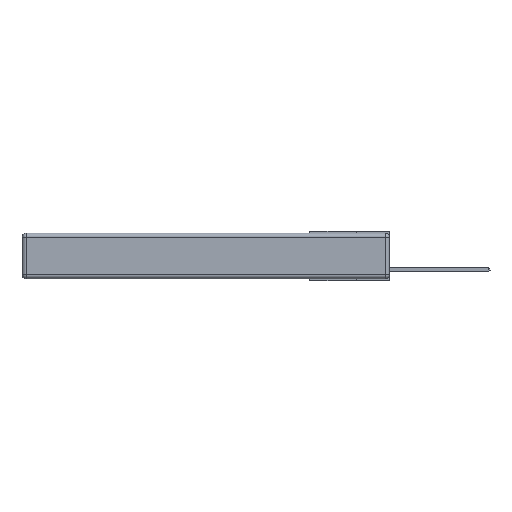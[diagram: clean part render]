
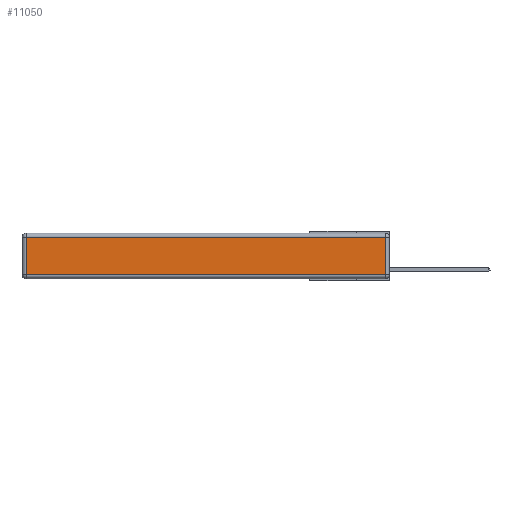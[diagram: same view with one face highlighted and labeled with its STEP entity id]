
A CAD part, left-side view. The second image highlights one B-rep face of the part: STEP entity #11050.
In plain terms, the highlighted planar face has unit normal (-1, 0, 0).
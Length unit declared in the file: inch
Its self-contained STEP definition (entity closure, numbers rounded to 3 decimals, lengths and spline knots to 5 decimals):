
#116 = LINE ( 'NONE', #6268, #12944 ) ;
#245 = CARTESIAN_POINT ( 'NONE',  ( 0., 0.03, -0.343 ) ) ;
#597 = CARTESIAN_POINT ( 'NONE',  ( 0., 2.72, -0.343 ) ) ;
#853 = ORIENTED_EDGE ( 'NONE', *, *, #5311, .T. ) ;
#2305 = LINE ( 'NONE', #245, #13569 ) ;
#3360 = DIRECTION ( 'NONE',  ( 0., -1., 0. ) ) ;
#3393 = VECTOR ( 'NONE', #10347, 39.37008 ) ;
#3435 = VERTEX_POINT ( 'NONE', #4758 ) ;
#3971 = DIRECTION ( 'NONE',  ( 0., 1., 0. ) ) ;
#4338 = FACE_OUTER_BOUND ( 'NONE', #10212, .T. ) ;
#4433 = EDGE_CURVE ( 'NONE', #3435, #5836, #9864, .T. ) ;
#4637 = EDGE_CURVE ( 'NONE', #13343, #3435, #116, .T. ) ;
#4758 = CARTESIAN_POINT ( 'NONE',  ( 0., 2.72, -0.03 ) ) ;
#4853 = ORIENTED_EDGE ( 'NONE', *, *, #4433, .T. ) ;
#5311 = EDGE_CURVE ( 'NONE', #5836, #13893, #11570, .T. ) ;
#5559 = CARTESIAN_POINT ( 'NONE',  ( 0., 0., -0.313 ) ) ;
#5647 = CARTESIAN_POINT ( 'NONE',  ( 0., 0.03, -0.313 ) ) ;
#5735 = ORIENTED_EDGE ( 'NONE', *, *, #11070, .T. ) ;
#5836 = VERTEX_POINT ( 'NONE', #12527 ) ;
#6268 = CARTESIAN_POINT ( 'NONE',  ( 0., 2.75, -0.03 ) ) ;
#6871 = PLANE ( 'NONE',  #13316 ) ;
#8672 = VECTOR ( 'NONE', #3360, 39.37008 ) ;
#9864 = LINE ( 'NONE', #597, #3393 ) ;
#10040 = DIRECTION ( 'NONE',  ( 0., 0., 1. ) ) ;
#10187 = DIRECTION ( 'NONE',  ( -1., 0., 0. ) ) ;
#10212 = EDGE_LOOP ( 'NONE', ( #853, #5735, #13121, #4853 ) ) ;
#10347 = DIRECTION ( 'NONE',  ( 0., 0., -1. ) ) ;
#11050 = ADVANCED_FACE ( 'NONE', ( #4338 ), #6871, .T. ) ;
#11070 = EDGE_CURVE ( 'NONE', #13893, #13343, #2305, .T. ) ;
#11088 = DIRECTION ( 'NONE',  ( 0., 0., 1. ) ) ;
#11570 = LINE ( 'NONE', #5559, #8672 ) ;
#12245 = CARTESIAN_POINT ( 'NONE',  ( 0., 0., -0.343 ) ) ;
#12527 = CARTESIAN_POINT ( 'NONE',  ( 0., 2.72, -0.313 ) ) ;
#12944 = VECTOR ( 'NONE', #3971, 39.37008 ) ;
#13121 = ORIENTED_EDGE ( 'NONE', *, *, #4637, .T. ) ;
#13316 = AXIS2_PLACEMENT_3D ( 'NONE', #12245, #10187, #10040 ) ;
#13343 = VERTEX_POINT ( 'NONE', #13469 ) ;
#13469 = CARTESIAN_POINT ( 'NONE',  ( 0., 0.03, -0.03 ) ) ;
#13569 = VECTOR ( 'NONE', #11088, 39.37008 ) ;
#13893 = VERTEX_POINT ( 'NONE', #5647 ) ;
